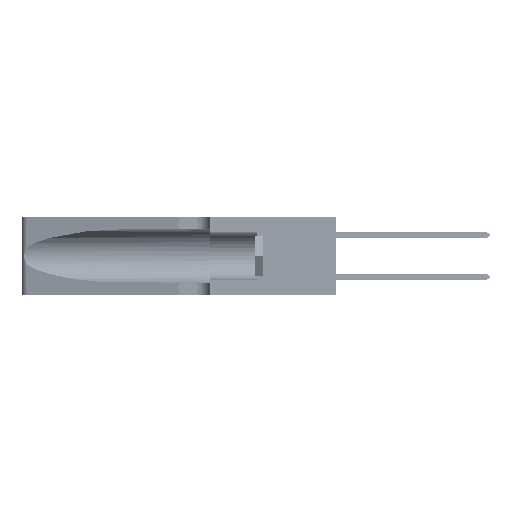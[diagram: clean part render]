
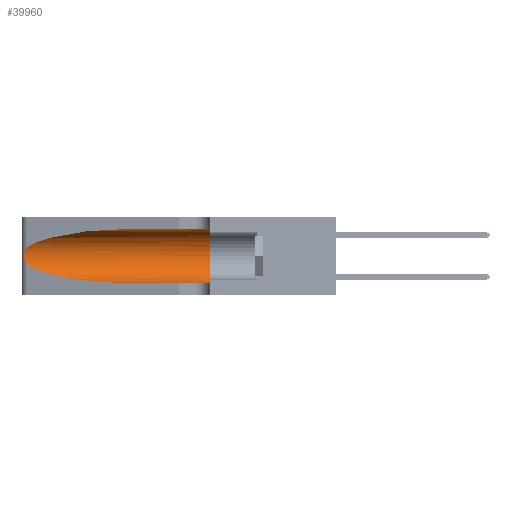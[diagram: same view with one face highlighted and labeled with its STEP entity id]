
A CAD part, left-side view. The second image highlights one B-rep face of the part: STEP entity #39960.
In plain terms, the highlighted cylindrical face has radius 3.308 mm (diameter 6.617 mm), a partial arc.
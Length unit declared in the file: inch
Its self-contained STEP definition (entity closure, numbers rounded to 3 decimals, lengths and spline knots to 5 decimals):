
#210 = ORIENTED_EDGE ( 'NONE', *, *, #16909, .T. ) ;
#464 = CARTESIAN_POINT ( 'NONE',  ( 0.1305, 0.72297, 0.05475 ) ) ;
#665 = EDGE_LOOP ( 'NONE', ( #11854, #210, #10955, #3336, #14132, #14466 ) ) ;
#2428 = CARTESIAN_POINT ( 'NONE',  ( 0.26017, 1.23833, 0.17102 ) ) ;
#3336 = ORIENTED_EDGE ( 'NONE', *, *, #3404, .T. ) ;
#3404 = EDGE_CURVE ( 'NONE', #6989, #39176, #22565, .T. ) ;
#6064 = DIRECTION ( 'NONE',  ( 0., 1., 0. ) ) ;
#6504 = CARTESIAN_POINT ( 'NONE',  ( 0.25789, 1.23486, 0.15765 ) ) ;
#6989 = VERTEX_POINT ( 'NONE', #464 ) ;
#10425 = CARTESIAN_POINT ( 'NONE',  ( 0.25487, 1.22718, 0.22369 ) ) ;
#10472 = EDGE_CURVE ( 'NONE', #31571, #6989, #42093, .T. ) ;
#10608 = CARTESIAN_POINT ( 'NONE',  ( 0.25555, 1.22993, 0.14849 ) ) ;
#10712 = CARTESIAN_POINT ( 'NONE',  ( 0.1305, 0.72297, 0.31525 ) ) ;
#10955 = ORIENTED_EDGE ( 'NONE', *, *, #10472, .T. ) ;
#11854 = ORIENTED_EDGE ( 'NONE', *, *, #31188, .T. ) ;
#14132 = ORIENTED_EDGE ( 'NONE', *, *, #19588, .F. ) ;
#14444 = CARTESIAN_POINT ( 'NONE',  ( 0.25555, 1.22994, 0.2215 ) ) ;
#14466 = ORIENTED_EDGE ( 'NONE', *, *, #32444, .F. ) ;
#14613 = B_SPLINE_CURVE_WITH_KNOTS ( 'NONE', 3,
 ( #10425, #14444, #42011, #18410, #45989, #22442, #49928, #26412, #2428, #30419, #6504, #34355, #10608, #38240 ),
 .UNSPECIFIED., .F., .F.,
 ( 4, 2, 2, 2, 2, 2, 4 ),
 ( 0., 0.00027, 0.00053, 0.00107, 0.0016, 0.00187, 0.00214 ),
 .UNSPECIFIED. ) ;
#14973 = CARTESIAN_POINT ( 'NONE',  ( 0.25487, 1.22718, 0.14631 ) ) ;
#16909 = EDGE_CURVE ( 'NONE', #48783, #31571, #14613, .T. ) ;
#18410 = CARTESIAN_POINT ( 'NONE',  ( 0.25787, 1.23484, 0.2124 ) ) ;
#18956 = CARTESIAN_POINT ( 'NONE',  ( 0.18966, 0.96281, 0.05475 ) ) ;
#19099 = CARTESIAN_POINT ( 'NONE',  ( 0.1305, 1.61858, 0.185 ) ) ;
#19588 = EDGE_CURVE ( 'NONE', #34505, #39176, #35699, .T. ) ;
#22442 = CARTESIAN_POINT ( 'NONE',  ( 0.26018, 1.23835, 0.19895 ) ) ;
#22565 = LINE ( 'NONE', #35881, #28113 ) ;
#22732 = CARTESIAN_POINT ( 'NONE',  ( 0.2373, 1.15595, 0.28018 ) ) ;
#22813 = CARTESIAN_POINT ( 'NONE',  ( 0.2373, 1.15595, 0.08982 ) ) ;
#23573 = AXIS2_PLACEMENT_3D ( 'NONE', #19099, #46657, #42679 ) ;
#24509 = LINE ( 'NONE', #41305, #32527 ) ;
#24593 = CARTESIAN_POINT ( 'NONE',  ( 0.25487, 1.22718, 0.14631 ) ) ;
#26412 = CARTESIAN_POINT ( 'NONE',  ( 0.26075, 1.23896, 0.178 ) ) ;
#28113 = VECTOR ( 'NONE', #39785, 39.37008 ) ;
#29972 = CARTESIAN_POINT ( 'NONE',  ( 0.1305, 0.35, 0.185 ) ) ;
#30419 = CARTESIAN_POINT ( 'NONE',  ( 0.25856, 1.23593, 0.16098 ) ) ;
#31188 = EDGE_CURVE ( 'NONE', #42086, #48783, #38336, .T. ) ;
#31571 = VERTEX_POINT ( 'NONE', #24593 ) ;
#32444 = EDGE_CURVE ( 'NONE', #42086, #34505, #24509, .T. ) ;
#32527 = VECTOR ( 'NONE', #45288, 39.37008 ) ;
#32629 = CYLINDRICAL_SURFACE ( 'NONE', #23573, 0.13025 ) ;
#32889 = CARTESIAN_POINT ( 'NONE',  ( 0.1305, 0.35, 0.31525 ) ) ;
#33920 = DIRECTION ( 'NONE',  ( 0., 0., 1. ) ) ;
#34355 = CARTESIAN_POINT ( 'NONE',  ( 0.25639, 1.23186, 0.15144 ) ) ;
#34505 = VERTEX_POINT ( 'NONE', #32889 ) ;
#35699 = CIRCLE ( 'NONE', #47311, 0.13025 ) ;
#35881 = CARTESIAN_POINT ( 'NONE',  ( 0.1305, 1.61858, 0.05475 ) ) ;
#38240 = CARTESIAN_POINT ( 'NONE',  ( 0.25487, 1.22718, 0.14631 ) ) ;
#38336 =( BOUNDED_CURVE ( )  B_SPLINE_CURVE ( 3, ( #10712, #42281, #22732, #50209 ),
 .UNSPECIFIED., .F., .F. ) 
 B_SPLINE_CURVE_WITH_KNOTS ( ( 4, 4 ),
 ( 1.5708, 2.84003 ),
 .UNSPECIFIED. ) 
 CURVE ( )  GEOMETRIC_REPRESENTATION_ITEM ( )  RATIONAL_B_SPLINE_CURVE ( ( 1., 0.87, 0.87, 1. ) ) 
 REPRESENTATION_ITEM ( '' )  );
#39176 = VERTEX_POINT ( 'NONE', #41022 ) ;
#39785 = DIRECTION ( 'NONE',  ( 0., -1., 0. ) ) ;
#39960 = ADVANCED_FACE ( 'NONE', ( #44277 ), #32629, .F. ) ;
#40630 = CARTESIAN_POINT ( 'NONE',  ( 0.1305, 0.72297, 0.31525 ) ) ;
#41022 = CARTESIAN_POINT ( 'NONE',  ( 0.1305, 0.35, 0.05475 ) ) ;
#41305 = CARTESIAN_POINT ( 'NONE',  ( 0.1305, 1.61858, 0.31525 ) ) ;
#42011 = CARTESIAN_POINT ( 'NONE',  ( 0.25639, 1.23184, 0.21858 ) ) ;
#42086 = VERTEX_POINT ( 'NONE', #40630 ) ;
#42093 =( BOUNDED_CURVE ( )  B_SPLINE_CURVE ( 3, ( #14973, #22813, #18956, #46521 ),
 .UNSPECIFIED., .F., .T. ) 
 B_SPLINE_CURVE_WITH_KNOTS ( ( 4, 4 ),
 ( 3.44316, 4.71239 ),
 .UNSPECIFIED. ) 
 CURVE ( )  GEOMETRIC_REPRESENTATION_ITEM ( )  RATIONAL_B_SPLINE_CURVE ( ( 1., 0.87, 0.87, 1. ) ) 
 REPRESENTATION_ITEM ( '' )  );
#42281 = CARTESIAN_POINT ( 'NONE',  ( 0.18966, 0.96281, 0.31525 ) ) ;
#42679 = DIRECTION ( 'NONE',  ( 0., 0., -1. ) ) ;
#44277 = FACE_OUTER_BOUND ( 'NONE', #665, .T. ) ;
#45288 = DIRECTION ( 'NONE',  ( 0., -1., 0. ) ) ;
#45989 = CARTESIAN_POINT ( 'NONE',  ( 0.25854, 1.2359, 0.20912 ) ) ;
#46521 = CARTESIAN_POINT ( 'NONE',  ( 0.1305, 0.72297, 0.05475 ) ) ;
#46657 = DIRECTION ( 'NONE',  ( 0., -1., 0. ) ) ;
#47311 = AXIS2_PLACEMENT_3D ( 'NONE', #29972, #6064, #33920 ) ;
#48783 = VERTEX_POINT ( 'NONE', #50055 ) ;
#49928 = CARTESIAN_POINT ( 'NONE',  ( 0.26075, 1.23896, 0.19203 ) ) ;
#50055 = CARTESIAN_POINT ( 'NONE',  ( 0.25487, 1.22718, 0.22369 ) ) ;
#50209 = CARTESIAN_POINT ( 'NONE',  ( 0.25487, 1.22718, 0.22369 ) ) ;
